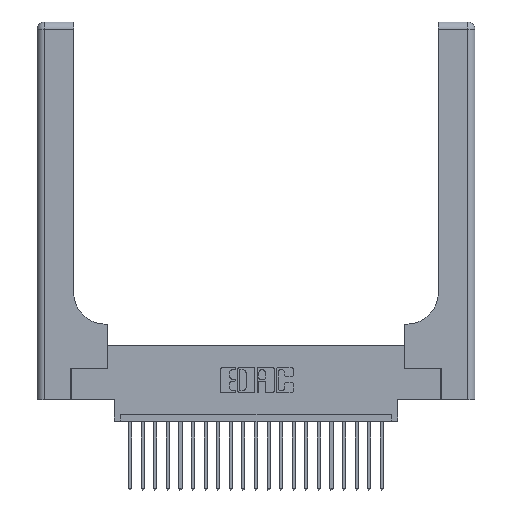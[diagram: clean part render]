
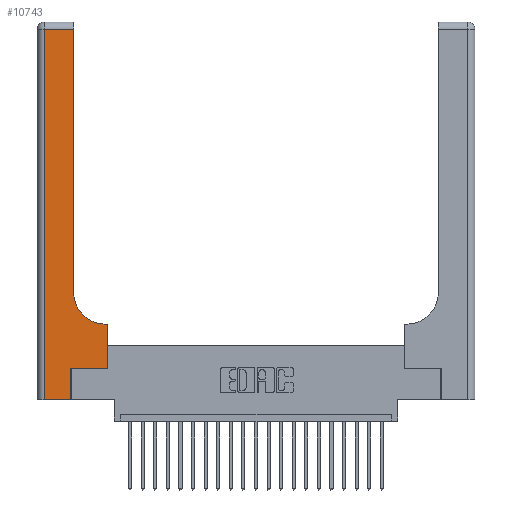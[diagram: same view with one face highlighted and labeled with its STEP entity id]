
A CAD part, top view. The second image highlights one B-rep face of the part: STEP entity #10743.
In plain terms, the highlighted planar face has unit normal (0, 0, 1).
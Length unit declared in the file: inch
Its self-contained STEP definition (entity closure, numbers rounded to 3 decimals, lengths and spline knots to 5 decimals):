
#230 = CARTESIAN_POINT ( 'NONE',  ( 0., 2.94, 0.37 ) ) ;
#469 = LINE ( 'NONE', #22342, #19833 ) ;
#472 = DIRECTION ( 'NONE',  ( 0., 0., -1. ) ) ;
#958 = CARTESIAN_POINT ( 'NONE',  ( 0., 0., 0.37 ) ) ;
#1263 = VERTEX_POINT ( 'NONE', #20164 ) ;
#1371 = CARTESIAN_POINT ( 'NONE',  ( 0.269, 0., 0.37 ) ) ;
#1510 = ORIENTED_EDGE ( 'NONE', *, *, #4080, .T. ) ;
#2221 = CARTESIAN_POINT ( 'NONE',  ( 0.5415, 0.85, 0.37 ) ) ;
#2503 = ORIENTED_EDGE ( 'NONE', *, *, #7293, .T. ) ;
#2544 = VECTOR ( 'NONE', #18131, 39.37008 ) ;
#3226 = VERTEX_POINT ( 'NONE', #9887 ) ;
#3326 = AXIS2_PLACEMENT_3D ( 'NONE', #2221, #472, #14962 ) ;
#4080 = EDGE_CURVE ( 'NONE', #1263, #23036, #16245, .T. ) ;
#4197 = EDGE_CURVE ( 'NONE', #18678, #21342, #7832, .T. ) ;
#4487 = CIRCLE ( 'NONE', #3326, 0.25 ) ;
#4726 = VECTOR ( 'NONE', #10937, 39.37008 ) ;
#4801 = EDGE_CURVE ( 'NONE', #7275, #15519, #6589, .T. ) ;
#5042 = VERTEX_POINT ( 'NONE', #20898 ) ;
#5294 = CARTESIAN_POINT ( 'NONE',  ( 0.269, 0.25, 0.37 ) ) ;
#5528 = AXIS2_PLACEMENT_3D ( 'NONE', #17148, #13440, #9763 ) ;
#5773 = DIRECTION ( 'NONE',  ( -1., 0., 0. ) ) ;
#5813 = LINE ( 'NONE', #230, #23506 ) ;
#6322 = FACE_OUTER_BOUND ( 'NONE', #16418, .T. ) ;
#6589 = LINE ( 'NONE', #18210, #2544 ) ;
#6894 = ORIENTED_EDGE ( 'NONE', *, *, #13138, .T. ) ;
#6964 = CARTESIAN_POINT ( 'NONE',  ( 0.5585, 0.25, 0.37 ) ) ;
#7094 = ORIENTED_EDGE ( 'NONE', *, *, #16862, .T. ) ;
#7215 = CARTESIAN_POINT ( 'NONE',  ( 0.269, 0., 0.37 ) ) ;
#7275 = VERTEX_POINT ( 'NONE', #12825 ) ;
#7293 = EDGE_CURVE ( 'NONE', #21342, #1263, #7588, .T. ) ;
#7561 = DIRECTION ( 'NONE',  ( 0., 1., 0. ) ) ;
#7588 = LINE ( 'NONE', #5294, #4726 ) ;
#7604 = CARTESIAN_POINT ( 'NONE',  ( 0.2915, 0.6, 0.37 ) ) ;
#7832 = LINE ( 'NONE', #1371, #15674 ) ;
#9290 = VECTOR ( 'NONE', #13550, 39.37008 ) ;
#9763 = DIRECTION ( 'NONE',  ( -1., 0., 0. ) ) ;
#9887 = CARTESIAN_POINT ( 'NONE',  ( 0.2915, 0.85, 0.37 ) ) ;
#10527 = DIRECTION ( 'NONE',  ( 0., 1., 0. ) ) ;
#10689 = CARTESIAN_POINT ( 'NONE',  ( 0.269, 0.25, 0.37 ) ) ;
#10743 = ADVANCED_FACE ( 'NONE', ( #6322 ), #19098, .F. ) ;
#10937 = DIRECTION ( 'NONE',  ( 1., 0., 0. ) ) ;
#12814 = EDGE_CURVE ( 'NONE', #23036, #5042, #15976, .T. ) ;
#12825 = CARTESIAN_POINT ( 'NONE',  ( 0.06, 2.94, 0.37 ) ) ;
#13138 = EDGE_CURVE ( 'NONE', #19730, #7275, #5813, .T. ) ;
#13145 = DIRECTION ( 'NONE',  ( -1., 0., 0. ) ) ;
#13440 = DIRECTION ( 'NONE',  ( 0., 0., -1. ) ) ;
#13550 = DIRECTION ( 'NONE',  ( 1., 0., 0. ) ) ;
#13563 = ORIENTED_EDGE ( 'NONE', *, *, #4197, .T. ) ;
#14811 = CARTESIAN_POINT ( 'NONE',  ( 0.06, 0., 0.37 ) ) ;
#14962 = DIRECTION ( 'NONE',  ( 1., 0., 0. ) ) ;
#15075 = ORIENTED_EDGE ( 'NONE', *, *, #16424, .T. ) ;
#15519 = VERTEX_POINT ( 'NONE', #14811 ) ;
#15674 = VECTOR ( 'NONE', #10527, 39.37008 ) ;
#15970 = CARTESIAN_POINT ( 'NONE',  ( 0.5585, 0.6, 0.37 ) ) ;
#15976 = LINE ( 'NONE', #7604, #23266 ) ;
#16245 = LINE ( 'NONE', #6964, #20337 ) ;
#16418 = EDGE_LOOP ( 'NONE', ( #7094, #6894, #16462, #22655, #13563, #2503, #1510, #18917, #15075 ) ) ;
#16424 = EDGE_CURVE ( 'NONE', #5042, #3226, #4487, .T. ) ;
#16462 = ORIENTED_EDGE ( 'NONE', *, *, #4801, .T. ) ;
#16642 = CARTESIAN_POINT ( 'NONE',  ( 0.2915, 2.94, 0.37 ) ) ;
#16862 = EDGE_CURVE ( 'NONE', #3226, #19730, #469, .T. ) ;
#17148 = CARTESIAN_POINT ( 'NONE',  ( 0., 3., 0.37 ) ) ;
#18131 = DIRECTION ( 'NONE',  ( 0., -1., 0. ) ) ;
#18210 = CARTESIAN_POINT ( 'NONE',  ( 0.06, 3., 0.37 ) ) ;
#18678 = VERTEX_POINT ( 'NONE', #7215 ) ;
#18917 = ORIENTED_EDGE ( 'NONE', *, *, #12814, .T. ) ;
#19098 = PLANE ( 'NONE',  #5528 ) ;
#19176 = LINE ( 'NONE', #958, #9290 ) ;
#19730 = VERTEX_POINT ( 'NONE', #16642 ) ;
#19833 = VECTOR ( 'NONE', #7561, 39.37008 ) ;
#20164 = CARTESIAN_POINT ( 'NONE',  ( 0.5585, 0.25, 0.37 ) ) ;
#20337 = VECTOR ( 'NONE', #21823, 39.37008 ) ;
#20898 = CARTESIAN_POINT ( 'NONE',  ( 0.5415, 0.6, 0.37 ) ) ;
#21147 = EDGE_CURVE ( 'NONE', #15519, #18678, #19176, .T. ) ;
#21342 = VERTEX_POINT ( 'NONE', #10689 ) ;
#21823 = DIRECTION ( 'NONE',  ( 0., 1., 0. ) ) ;
#22342 = CARTESIAN_POINT ( 'NONE',  ( 0.2915, 3., 0.37 ) ) ;
#22655 = ORIENTED_EDGE ( 'NONE', *, *, #21147, .T. ) ;
#23036 = VERTEX_POINT ( 'NONE', #15970 ) ;
#23266 = VECTOR ( 'NONE', #13145, 39.37008 ) ;
#23506 = VECTOR ( 'NONE', #5773, 39.37008 ) ;
